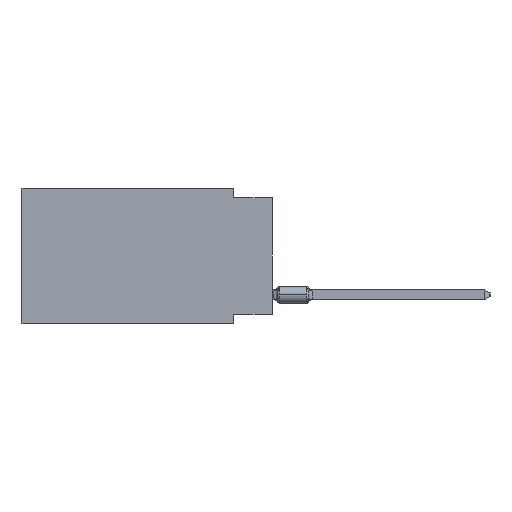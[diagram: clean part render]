
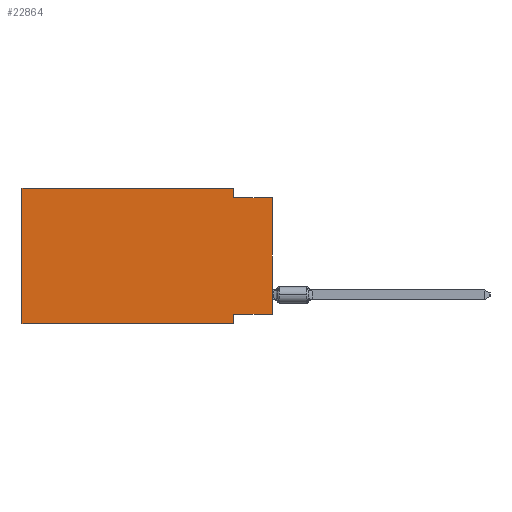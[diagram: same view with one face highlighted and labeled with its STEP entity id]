
A CAD part, left-side view. The second image highlights one B-rep face of the part: STEP entity #22864.
In plain terms, the highlighted planar face has unit normal (-1, 0, 0).
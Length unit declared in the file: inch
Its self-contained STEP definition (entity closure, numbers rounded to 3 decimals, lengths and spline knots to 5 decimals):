
#171 = ORIENTED_EDGE ( 'NONE', *, *, #18800, .F. ) ;
#191 = DIRECTION ( 'NONE',  ( 0., 1., 0. ) ) ;
#249 = LINE ( 'NONE', #23540, #14445 ) ;
#525 = CARTESIAN_POINT ( 'NONE',  ( 0., 0.645, -0.35 ) ) ;
#1435 = VECTOR ( 'NONE', #2200, 39.37008 ) ;
#1605 = ORIENTED_EDGE ( 'NONE', *, *, #16251, .F. ) ;
#1758 = VERTEX_POINT ( 'NONE', #16703 ) ;
#2190 = LINE ( 'NONE', #2337, #15747 ) ;
#2200 = DIRECTION ( 'NONE',  ( 0., 0., -1. ) ) ;
#2227 = LINE ( 'NONE', #15974, #17597 ) ;
#2337 = CARTESIAN_POINT ( 'NONE',  ( 0., 0., 0. ) ) ;
#2373 = DIRECTION ( 'NONE',  ( 0., 0., 1. ) ) ;
#2442 = VECTOR ( 'NONE', #191, 39.37008 ) ;
#4020 = VERTEX_POINT ( 'NONE', #20049 ) ;
#4053 = LINE ( 'NONE', #18577, #1435 ) ;
#4193 = ORIENTED_EDGE ( 'NONE', *, *, #26444, .F. ) ;
#4338 = VERTEX_POINT ( 'NONE', #4896 ) ;
#4604 = CARTESIAN_POINT ( 'NONE',  ( 0., 0.1, -0.025 ) ) ;
#4837 = VERTEX_POINT ( 'NONE', #14896 ) ;
#4896 = CARTESIAN_POINT ( 'NONE',  ( 0., 0., -0.325 ) ) ;
#4899 = LINE ( 'NONE', #10142, #23231 ) ;
#6734 = DIRECTION ( 'NONE',  ( 0., -1., 0. ) ) ;
#6864 = DIRECTION ( 'NONE',  ( 1., 0., 0. ) ) ;
#7788 = CARTESIAN_POINT ( 'NONE',  ( 0., 0.645, 0. ) ) ;
#9191 = CARTESIAN_POINT ( 'NONE',  ( 0., 0.645, 0. ) ) ;
#9596 = VERTEX_POINT ( 'NONE', #4604 ) ;
#9743 = DIRECTION ( 'NONE',  ( 0., 0., -1. ) ) ;
#10142 = CARTESIAN_POINT ( 'NONE',  ( 0., 0.645, 0. ) ) ;
#10945 = CARTESIAN_POINT ( 'NONE',  ( 0., 0.1, 0. ) ) ;
#11604 = DIRECTION ( 'NONE',  ( 0., 0., 1. ) ) ;
#12461 = DIRECTION ( 'NONE',  ( 0., -1., 0. ) ) ;
#13038 = DIRECTION ( 'NONE',  ( 0., -1., 0. ) ) ;
#14445 = VECTOR ( 'NONE', #6734, 39.37008 ) ;
#14824 = ORIENTED_EDGE ( 'NONE', *, *, #20096, .F. ) ;
#14896 = CARTESIAN_POINT ( 'NONE',  ( 0., 0.1, -0.325 ) ) ;
#15445 = VERTEX_POINT ( 'NONE', #10945 ) ;
#15644 = VECTOR ( 'NONE', #9743, 39.37008 ) ;
#15747 = VECTOR ( 'NONE', #11604, 39.37008 ) ;
#15974 = CARTESIAN_POINT ( 'NONE',  ( 0., 0.645, 0. ) ) ;
#16144 = EDGE_CURVE ( 'NONE', #30510, #1758, #17374, .T. ) ;
#16251 = EDGE_CURVE ( 'NONE', #4837, #1758, #19020, .T. ) ;
#16703 = CARTESIAN_POINT ( 'NONE',  ( 0., 0.1, -0.35 ) ) ;
#17374 = LINE ( 'NONE', #22588, #18613 ) ;
#17597 = VECTOR ( 'NONE', #2373, 39.37008 ) ;
#18577 = CARTESIAN_POINT ( 'NONE',  ( 0., 0.1, 0. ) ) ;
#18609 = DIRECTION ( 'NONE',  ( 0., 0., -1. ) ) ;
#18613 = VECTOR ( 'NONE', #13038, 39.37008 ) ;
#18711 = LINE ( 'NONE', #19031, #2442 ) ;
#18790 = EDGE_CURVE ( 'NONE', #4338, #4020, #2190, .T. ) ;
#18800 = EDGE_CURVE ( 'NONE', #4338, #4837, #18711, .T. ) ;
#19020 = LINE ( 'NONE', #22744, #15644 ) ;
#19031 = CARTESIAN_POINT ( 'NONE',  ( 0., 0., -0.325 ) ) ;
#20049 = CARTESIAN_POINT ( 'NONE',  ( 0., 0., -0.025 ) ) ;
#20096 = EDGE_CURVE ( 'NONE', #9596, #4020, #249, .T. ) ;
#22588 = CARTESIAN_POINT ( 'NONE',  ( 0., 0.645, -0.35 ) ) ;
#22744 = CARTESIAN_POINT ( 'NONE',  ( 0., 0.1, -0.35 ) ) ;
#22864 = ADVANCED_FACE ( 'NONE', ( #30294 ), #25663, .F. ) ;
#23231 = VECTOR ( 'NONE', #12461, 39.37008 ) ;
#23540 = CARTESIAN_POINT ( 'NONE',  ( 0., 0., -0.025 ) ) ;
#23913 = AXIS2_PLACEMENT_3D ( 'NONE', #9191, #6864, #18609 ) ;
#24808 = EDGE_CURVE ( 'NONE', #30510, #27879, #2227, .T. ) ;
#25663 = PLANE ( 'NONE',  #23913 ) ;
#26109 = ORIENTED_EDGE ( 'NONE', *, *, #16144, .T. ) ;
#26444 = EDGE_CURVE ( 'NONE', #15445, #9596, #4053, .T. ) ;
#26474 = ORIENTED_EDGE ( 'NONE', *, *, #24808, .F. ) ;
#27583 = ORIENTED_EDGE ( 'NONE', *, *, #28990, .F. ) ;
#27879 = VERTEX_POINT ( 'NONE', #7788 ) ;
#28748 = EDGE_LOOP ( 'NONE', ( #29626, #14824, #4193, #27583, #26474, #26109, #1605, #171 ) ) ;
#28990 = EDGE_CURVE ( 'NONE', #27879, #15445, #4899, .T. ) ;
#29626 = ORIENTED_EDGE ( 'NONE', *, *, #18790, .T. ) ;
#30294 = FACE_OUTER_BOUND ( 'NONE', #28748, .T. ) ;
#30510 = VERTEX_POINT ( 'NONE', #525 ) ;
